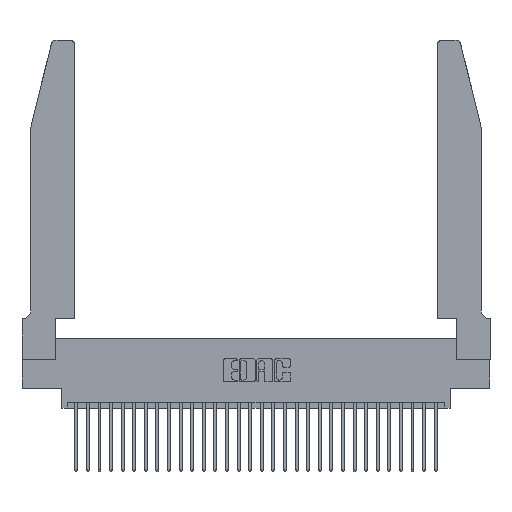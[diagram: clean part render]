
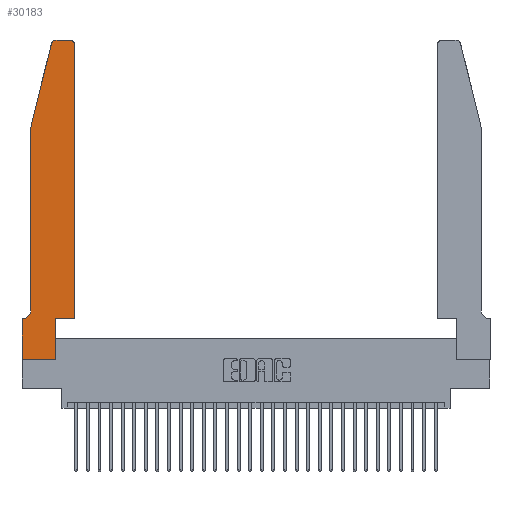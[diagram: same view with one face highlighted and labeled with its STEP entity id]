
A CAD part, top view. The second image highlights one B-rep face of the part: STEP entity #30183.
In plain terms, the highlighted planar face has unit normal (0, 0, 1).
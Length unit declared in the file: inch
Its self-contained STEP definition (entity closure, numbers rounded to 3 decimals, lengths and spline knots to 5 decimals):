
#222 = VECTOR ( 'NONE', #6272, 39.37008 ) ;
#346 = DIRECTION ( 'NONE',  ( 1., 0., 0. ) ) ;
#540 = CARTESIAN_POINT ( 'NONE',  ( 0.4505, 0.35, 0.37 ) ) ;
#1137 = CARTESIAN_POINT ( 'NONE',  ( 0.4505, 0.35, 0.37 ) ) ;
#1596 = VECTOR ( 'NONE', #31063, 39.37008 ) ;
#1904 = LINE ( 'NONE', #5736, #10009 ) ;
#1944 = VECTOR ( 'NONE', #3027, 39.37008 ) ;
#2920 = CARTESIAN_POINT ( 'NONE',  ( 0.4205, 2.72, 0.37 ) ) ;
#3027 = DIRECTION ( 'NONE',  ( 0., -1., 0. ) ) ;
#3288 = VERTEX_POINT ( 'NONE', #15235 ) ;
#3366 = VECTOR ( 'NONE', #27182, 39.37008 ) ;
#3377 = EDGE_CURVE ( 'NONE', #26207, #18096, #1904, .T. ) ;
#3831 = PLANE ( 'NONE',  #14692 ) ;
#4379 = EDGE_CURVE ( 'NONE', #27992, #5934, #26674, .T. ) ;
#5372 = DIRECTION ( 'NONE',  ( -1., 0., 0. ) ) ;
#5413 = DIRECTION ( 'NONE',  ( 1., 0., 0. ) ) ;
#5557 = DIRECTION ( 'NONE',  ( 0., 0., -1. ) ) ;
#5736 = CARTESIAN_POINT ( 'NONE',  ( 0.0755, 0.35, 0.37 ) ) ;
#5844 = EDGE_CURVE ( 'NONE', #18096, #21781, #15063, .T. ) ;
#5934 = VERTEX_POINT ( 'NONE', #30009 ) ;
#6272 = DIRECTION ( 'NONE',  ( 0., -1., 0. ) ) ;
#6325 = DIRECTION ( 'NONE',  ( 0., 0., 1. ) ) ;
#6586 = CARTESIAN_POINT ( 'NONE',  ( 0., 0., 0.37 ) ) ;
#6829 = EDGE_CURVE ( 'NONE', #26013, #9878, #12654, .T. ) ;
#6833 = DIRECTION ( 'NONE',  ( 0., 1., 0. ) ) ;
#6883 = LINE ( 'NONE', #6586, #19153 ) ;
#7302 = CARTESIAN_POINT ( 'NONE',  ( 0.2865, 0.35, 0.37 ) ) ;
#8668 = CIRCLE ( 'NONE', #26624, 0.03 ) ;
#9075 = DIRECTION ( 'NONE',  ( 1., 0., 0. ) ) ;
#9222 = CARTESIAN_POINT ( 'NONE',  ( 0.25487, 2.72718, 0.37 ) ) ;
#9246 = CARTESIAN_POINT ( 'NONE',  ( 0.2865, 0., 0.37 ) ) ;
#9594 = CARTESIAN_POINT ( 'NONE',  ( 0., 0., 0.37 ) ) ;
#9791 = DIRECTION ( 'NONE',  ( 0., 1., 0. ) ) ;
#9878 = VERTEX_POINT ( 'NONE', #12710 ) ;
#10009 = VECTOR ( 'NONE', #20372, 39.37008 ) ;
#10697 = VERTEX_POINT ( 'NONE', #9222 ) ;
#11232 = EDGE_CURVE ( 'NONE', #21781, #27992, #6883, .T. ) ;
#11634 = EDGE_LOOP ( 'NONE', ( #29775, #19821, #13263, #19380, #17253, #12329, #19524, #12925, #30070, #23531, #16535, #19594 ) ) ;
#11723 = CARTESIAN_POINT ( 'NONE',  ( 0.4505, 0.35, 0.37 ) ) ;
#12329 = ORIENTED_EDGE ( 'NONE', *, *, #3377, .T. ) ;
#12654 = LINE ( 'NONE', #11723, #13427 ) ;
#12710 = CARTESIAN_POINT ( 'NONE',  ( 0.4505, 2.72, 0.37 ) ) ;
#12888 = CARTESIAN_POINT ( 'NONE',  ( 0.284, 2.75, 0.37 ) ) ;
#12925 = ORIENTED_EDGE ( 'NONE', *, *, #11232, .T. ) ;
#13263 = ORIENTED_EDGE ( 'NONE', *, *, #21185, .T. ) ;
#13317 = VERTEX_POINT ( 'NONE', #21109 ) ;
#13319 = LINE ( 'NONE', #30545, #222 ) ;
#13427 = VECTOR ( 'NONE', #6833, 39.37008 ) ;
#13664 = CARTESIAN_POINT ( 'NONE',  ( 0., 0.35, 0.37 ) ) ;
#13797 = VERTEX_POINT ( 'NONE', #23256 ) ;
#13947 = VECTOR ( 'NONE', #9791, 39.37008 ) ;
#14477 = CARTESIAN_POINT ( 'NONE',  ( 0., 0.35, 0.37 ) ) ;
#14692 = AXIS2_PLACEMENT_3D ( 'NONE', #13664, #6325, #23336 ) ;
#15063 = LINE ( 'NONE', #24852, #1944 ) ;
#15126 = DIRECTION ( 'NONE',  ( 0., 0., 1. ) ) ;
#15164 = EDGE_CURVE ( 'NONE', #13317, #26207, #18919, .T. ) ;
#15235 = CARTESIAN_POINT ( 'NONE',  ( 0.0755, 2., 0.37 ) ) ;
#15581 = LINE ( 'NONE', #20026, #28242 ) ;
#16535 = ORIENTED_EDGE ( 'NONE', *, *, #6829, .T. ) ;
#16669 = AXIS2_PLACEMENT_3D ( 'NONE', #29392, #15126, #346 ) ;
#17253 = ORIENTED_EDGE ( 'NONE', *, *, #15164, .T. ) ;
#17922 = EDGE_CURVE ( 'NONE', #3288, #13317, #13319, .T. ) ;
#18096 = VERTEX_POINT ( 'NONE', #14477 ) ;
#18919 = CIRCLE ( 'NONE', #20522, 0.07 ) ;
#19153 = VECTOR ( 'NONE', #9075, 39.37008 ) ;
#19161 = CARTESIAN_POINT ( 'NONE',  ( 0.0055, 0.35, 0.37 ) ) ;
#19380 = ORIENTED_EDGE ( 'NONE', *, *, #17922, .T. ) ;
#19524 = ORIENTED_EDGE ( 'NONE', *, *, #5844, .T. ) ;
#19594 = ORIENTED_EDGE ( 'NONE', *, *, #26987, .T. ) ;
#19821 = ORIENTED_EDGE ( 'NONE', *, *, #28893, .T. ) ;
#20011 = CIRCLE ( 'NONE', #16669, 0.03 ) ;
#20026 = CARTESIAN_POINT ( 'NONE',  ( 0.2605, 2.75, 0.37 ) ) ;
#20064 = DIRECTION ( 'NONE',  ( 0., 0., 1. ) ) ;
#20187 = CARTESIAN_POINT ( 'NONE',  ( 0.0055, 0.42, 0.37 ) ) ;
#20372 = DIRECTION ( 'NONE',  ( -1., 0., 0. ) ) ;
#20522 = AXIS2_PLACEMENT_3D ( 'NONE', #20187, #5557, #22594 ) ;
#21109 = CARTESIAN_POINT ( 'NONE',  ( 0.0755, 0.42, 0.37 ) ) ;
#21122 = LINE ( 'NONE', #28653, #1596 ) ;
#21185 = EDGE_CURVE ( 'NONE', #10697, #3288, #21122, .T. ) ;
#21781 = VERTEX_POINT ( 'NONE', #9594 ) ;
#22594 = DIRECTION ( 'NONE',  ( -1., 0., 0. ) ) ;
#23191 = EDGE_CURVE ( 'NONE', #5934, #26013, #28383, .T. ) ;
#23256 = CARTESIAN_POINT ( 'NONE',  ( 0.4205, 2.75, 0.37 ) ) ;
#23336 = DIRECTION ( 'NONE',  ( 1., 0., 0. ) ) ;
#23531 = ORIENTED_EDGE ( 'NONE', *, *, #23191, .T. ) ;
#24852 = CARTESIAN_POINT ( 'NONE',  ( 0., 0., 0.37 ) ) ;
#25114 = FACE_OUTER_BOUND ( 'NONE', #11634, .T. ) ;
#25828 = VERTEX_POINT ( 'NONE', #12888 ) ;
#26013 = VERTEX_POINT ( 'NONE', #1137 ) ;
#26207 = VERTEX_POINT ( 'NONE', #19161 ) ;
#26624 = AXIS2_PLACEMENT_3D ( 'NONE', #2920, #20064, #5413 ) ;
#26674 = LINE ( 'NONE', #7302, #13947 ) ;
#26987 = EDGE_CURVE ( 'NONE', #9878, #13797, #8668, .T. ) ;
#27182 = DIRECTION ( 'NONE',  ( 1., 0., 0. ) ) ;
#27599 = EDGE_CURVE ( 'NONE', #13797, #25828, #15581, .T. ) ;
#27992 = VERTEX_POINT ( 'NONE', #9246 ) ;
#28242 = VECTOR ( 'NONE', #5372, 39.37008 ) ;
#28383 = LINE ( 'NONE', #540, #3366 ) ;
#28653 = CARTESIAN_POINT ( 'NONE',  ( 0.0755, 2., 0.37 ) ) ;
#28893 = EDGE_CURVE ( 'NONE', #25828, #10697, #20011, .T. ) ;
#29392 = CARTESIAN_POINT ( 'NONE',  ( 0.284, 2.72, 0.37 ) ) ;
#29775 = ORIENTED_EDGE ( 'NONE', *, *, #27599, .T. ) ;
#30009 = CARTESIAN_POINT ( 'NONE',  ( 0.2865, 0.35, 0.37 ) ) ;
#30070 = ORIENTED_EDGE ( 'NONE', *, *, #4379, .T. ) ;
#30183 = ADVANCED_FACE ( 'NONE', ( #25114 ), #3831, .T. ) ;
#30545 = CARTESIAN_POINT ( 'NONE',  ( 0.0755, 2., 0.37 ) ) ;
#31063 = DIRECTION ( 'NONE',  ( -0.239, -0.971, 0. ) ) ;
